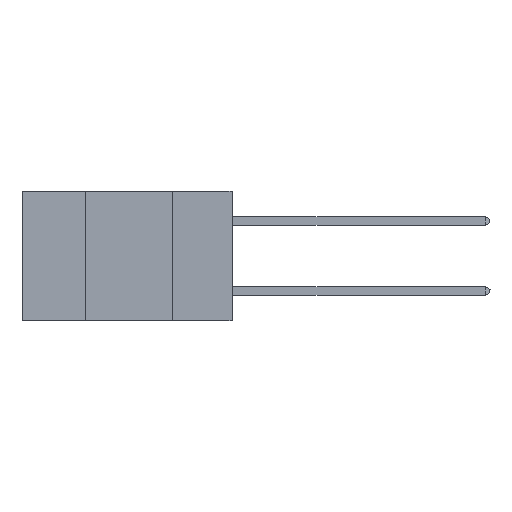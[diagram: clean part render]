
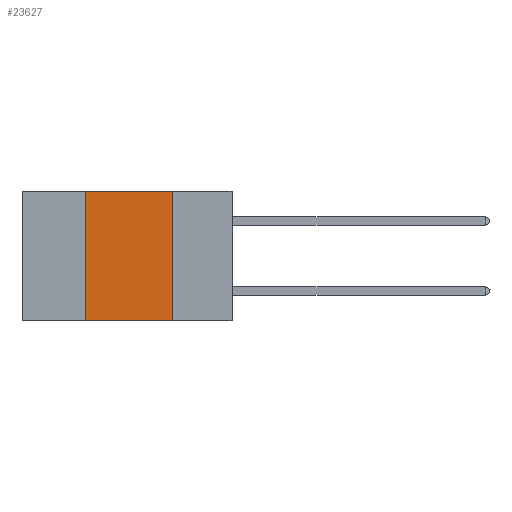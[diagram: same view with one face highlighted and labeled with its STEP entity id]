
A CAD part, left-side view. The second image highlights one B-rep face of the part: STEP entity #23627.
In plain terms, the highlighted planar face has unit normal (-1, 0, 0).
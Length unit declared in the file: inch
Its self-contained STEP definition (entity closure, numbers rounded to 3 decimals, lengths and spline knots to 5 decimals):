
#653 = ORIENTED_EDGE ( 'NONE', *, *, #17322, .F. ) ;
#1106 = VECTOR ( 'NONE', #23634, 39.37008 ) ;
#1152 = VERTEX_POINT ( 'NONE', #8879 ) ;
#1243 = DIRECTION ( 'NONE',  ( 0., 0., -1. ) ) ;
#1930 = EDGE_CURVE ( 'NONE', #12062, #1152, #5271, .T. ) ;
#2845 = EDGE_CURVE ( 'NONE', #13232, #9491, #8085, .T. ) ;
#3176 = PLANE ( 'NONE',  #11745 ) ;
#3272 = DIRECTION ( 'NONE',  ( 1., 0., 0. ) ) ;
#4706 = CARTESIAN_POINT ( 'NONE',  ( 0., 0.17, 0. ) ) ;
#5271 = LINE ( 'NONE', #7709, #14333 ) ;
#7709 = CARTESIAN_POINT ( 'NONE',  ( 0., 0.42, 0. ) ) ;
#8085 = LINE ( 'NONE', #18050, #23100 ) ;
#8879 = CARTESIAN_POINT ( 'NONE',  ( 0., 0.42, 0. ) ) ;
#9079 = ORIENTED_EDGE ( 'NONE', *, *, #15502, .T. ) ;
#9214 = EDGE_LOOP ( 'NONE', ( #25932, #653, #10246, #9079 ) ) ;
#9491 = VERTEX_POINT ( 'NONE', #17610 ) ;
#9783 = DIRECTION ( 'NONE',  ( 0., 0., 1. ) ) ;
#10246 = ORIENTED_EDGE ( 'NONE', *, *, #1930, .F. ) ;
#11745 = AXIS2_PLACEMENT_3D ( 'NONE', #19656, #3272, #1243 ) ;
#12062 = VERTEX_POINT ( 'NONE', #26047 ) ;
#12191 = DIRECTION ( 'NONE',  ( 0., 0., -1. ) ) ;
#13232 = VERTEX_POINT ( 'NONE', #4706 ) ;
#14333 = VECTOR ( 'NONE', #9783, 39.37008 ) ;
#15502 = EDGE_CURVE ( 'NONE', #12062, #9491, #17970, .T. ) ;
#15709 = VECTOR ( 'NONE', #20215, 39.37008 ) ;
#17322 = EDGE_CURVE ( 'NONE', #1152, #13232, #24161, .T. ) ;
#17610 = CARTESIAN_POINT ( 'NONE',  ( 0., 0.17, -0.37 ) ) ;
#17970 = LINE ( 'NONE', #26261, #15709 ) ;
#18050 = CARTESIAN_POINT ( 'NONE',  ( 0., 0.17, 0. ) ) ;
#19609 = CARTESIAN_POINT ( 'NONE',  ( 0., 0.6, 0. ) ) ;
#19656 = CARTESIAN_POINT ( 'NONE',  ( 0., 0.6, 0. ) ) ;
#20215 = DIRECTION ( 'NONE',  ( 0., -1., 0. ) ) ;
#23100 = VECTOR ( 'NONE', #12191, 39.37008 ) ;
#23627 = ADVANCED_FACE ( 'NONE', ( #24319 ), #3176, .F. ) ;
#23634 = DIRECTION ( 'NONE',  ( 0., -1., 0. ) ) ;
#24161 = LINE ( 'NONE', #19609, #1106 ) ;
#24319 = FACE_OUTER_BOUND ( 'NONE', #9214, .T. ) ;
#25932 = ORIENTED_EDGE ( 'NONE', *, *, #2845, .F. ) ;
#26047 = CARTESIAN_POINT ( 'NONE',  ( 0., 0.42, -0.37 ) ) ;
#26261 = CARTESIAN_POINT ( 'NONE',  ( 0., 0.6, -0.37 ) ) ;
